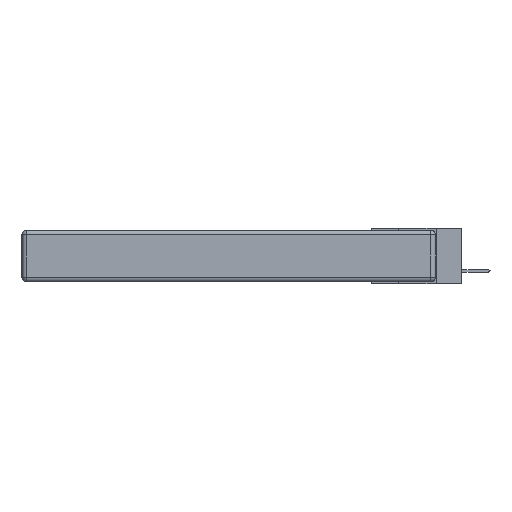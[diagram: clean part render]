
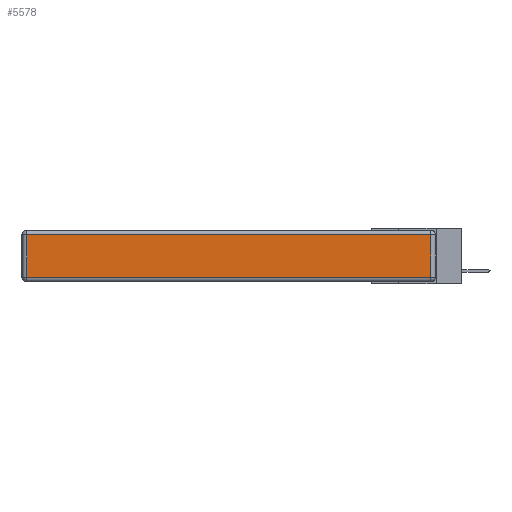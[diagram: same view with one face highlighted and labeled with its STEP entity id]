
A CAD part, left-side view. The second image highlights one B-rep face of the part: STEP entity #5578.
In plain terms, the highlighted planar face has unit normal (-1, 0, 0).
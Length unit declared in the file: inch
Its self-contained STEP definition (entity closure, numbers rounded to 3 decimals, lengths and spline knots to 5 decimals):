
#336 = CARTESIAN_POINT ( 'NONE',  ( 0., 0.03, -0.343 ) ) ;
#1184 = LINE ( 'NONE', #12985, #3667 ) ;
#1526 = EDGE_CURVE ( 'NONE', #2155, #14439, #7192, .T. ) ;
#1546 = CARTESIAN_POINT ( 'NONE',  ( 0., 2.72, -0.343 ) ) ;
#2155 = VERTEX_POINT ( 'NONE', #3427 ) ;
#2737 = CARTESIAN_POINT ( 'NONE',  ( 0., 0., -0.313 ) ) ;
#3427 = CARTESIAN_POINT ( 'NONE',  ( 0., 0.03, -0.313 ) ) ;
#3667 = VECTOR ( 'NONE', #17771, 39.37008 ) ;
#4040 = ORIENTED_EDGE ( 'NONE', *, *, #13882, .T. ) ;
#4354 = ORIENTED_EDGE ( 'NONE', *, *, #20093, .T. ) ;
#5528 = PLANE ( 'NONE',  #8151 ) ;
#5578 = ADVANCED_FACE ( 'NONE', ( #6203 ), #5528, .T. ) ;
#6203 = FACE_OUTER_BOUND ( 'NONE', #13396, .T. ) ;
#6456 = VECTOR ( 'NONE', #8656, 39.37008 ) ;
#7192 = LINE ( 'NONE', #336, #6456 ) ;
#7404 = DIRECTION ( 'NONE',  ( 0., -1., 0. ) ) ;
#7445 = ORIENTED_EDGE ( 'NONE', *, *, #1526, .T. ) ;
#8151 = AXIS2_PLACEMENT_3D ( 'NONE', #20140, #20075, #12152 ) ;
#8656 = DIRECTION ( 'NONE',  ( 0., 0., 1. ) ) ;
#8776 = VERTEX_POINT ( 'NONE', #18198 ) ;
#9461 = EDGE_CURVE ( 'NONE', #11446, #8776, #20735, .T. ) ;
#9835 = VECTOR ( 'NONE', #13014, 39.37008 ) ;
#11446 = VERTEX_POINT ( 'NONE', #12441 ) ;
#11919 = LINE ( 'NONE', #2737, #15409 ) ;
#12152 = DIRECTION ( 'NONE',  ( 0., 0., 1. ) ) ;
#12441 = CARTESIAN_POINT ( 'NONE',  ( 0., 2.72, -0.03 ) ) ;
#12965 = CARTESIAN_POINT ( 'NONE',  ( 0., 0.03, -0.03 ) ) ;
#12985 = CARTESIAN_POINT ( 'NONE',  ( 0., 2.75, -0.03 ) ) ;
#13014 = DIRECTION ( 'NONE',  ( 0., 0., -1. ) ) ;
#13396 = EDGE_LOOP ( 'NONE', ( #4354, #7445, #4040, #18666 ) ) ;
#13882 = EDGE_CURVE ( 'NONE', #14439, #11446, #1184, .T. ) ;
#14439 = VERTEX_POINT ( 'NONE', #12965 ) ;
#15409 = VECTOR ( 'NONE', #7404, 39.37008 ) ;
#17771 = DIRECTION ( 'NONE',  ( 0., 1., 0. ) ) ;
#18198 = CARTESIAN_POINT ( 'NONE',  ( 0., 2.72, -0.313 ) ) ;
#18666 = ORIENTED_EDGE ( 'NONE', *, *, #9461, .T. ) ;
#20075 = DIRECTION ( 'NONE',  ( -1., 0., 0. ) ) ;
#20093 = EDGE_CURVE ( 'NONE', #8776, #2155, #11919, .T. ) ;
#20140 = CARTESIAN_POINT ( 'NONE',  ( 0., 0., -0.343 ) ) ;
#20735 = LINE ( 'NONE', #1546, #9835 ) ;
